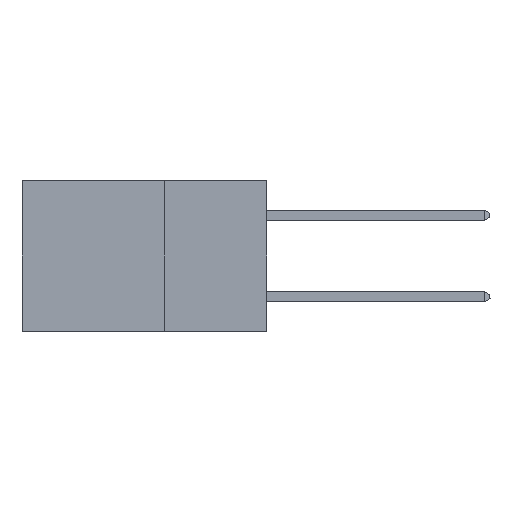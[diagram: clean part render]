
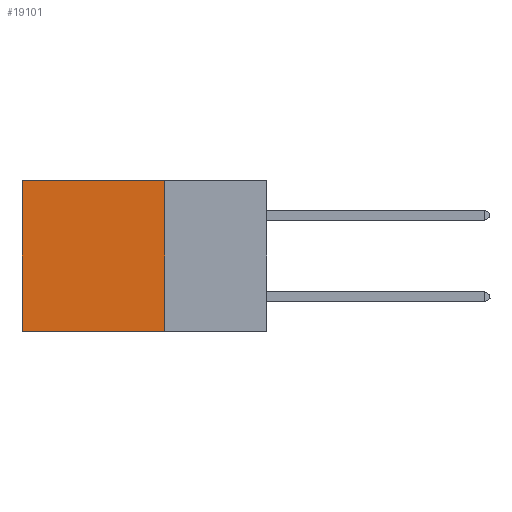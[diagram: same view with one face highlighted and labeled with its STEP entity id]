
A CAD part, left-side view. The second image highlights one B-rep face of the part: STEP entity #19101.
In plain terms, the highlighted planar face has unit normal (-1, 0, 0).
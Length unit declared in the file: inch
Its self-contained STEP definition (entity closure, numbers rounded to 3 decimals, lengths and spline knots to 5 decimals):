
#28 = DIRECTION ( 'NONE',  ( 0., 1., 0. ) ) ;
#558 = ORIENTED_EDGE ( 'NONE', *, *, #1156, .T. ) ;
#1156 = EDGE_CURVE ( 'NONE', #19799, #18990, #14665, .T. ) ;
#2888 = CARTESIAN_POINT ( 'NONE',  ( 0.2875, 0.25, 0. ) ) ;
#3376 = DIRECTION ( 'NONE',  ( 0., 1., 0. ) ) ;
#3559 = CARTESIAN_POINT ( 'NONE',  ( 0.2875, 0.25, 0. ) ) ;
#3904 = VECTOR ( 'NONE', #14393, 39.37008 ) ;
#3976 = VECTOR ( 'NONE', #3376, 39.37008 ) ;
#7139 = ORIENTED_EDGE ( 'NONE', *, *, #22710, .T. ) ;
#7356 = CARTESIAN_POINT ( 'NONE',  ( 0.2875, 0.6, -0.37 ) ) ;
#7572 = AXIS2_PLACEMENT_3D ( 'NONE', #2888, #20897, #8962 ) ;
#8962 = DIRECTION ( 'NONE',  ( 0., 0., -1. ) ) ;
#10166 = EDGE_LOOP ( 'NONE', ( #7139, #22189, #18478, #558 ) ) ;
#11651 = DIRECTION ( 'NONE',  ( 0., 0., -1. ) ) ;
#12366 = CARTESIAN_POINT ( 'NONE',  ( 0.2875, 0.6, 0. ) ) ;
#14393 = DIRECTION ( 'NONE',  ( 0., 0., -1. ) ) ;
#14583 = LINE ( 'NONE', #21524, #19847 ) ;
#14604 = CARTESIAN_POINT ( 'NONE',  ( 0.2875, 0.6, 0. ) ) ;
#14665 = LINE ( 'NONE', #3559, #3976 ) ;
#14935 = PLANE ( 'NONE',  #7572 ) ;
#15094 = VERTEX_POINT ( 'NONE', #7356 ) ;
#16338 = FACE_OUTER_BOUND ( 'NONE', #10166, .T. ) ;
#16827 = VERTEX_POINT ( 'NONE', #25255 ) ;
#16915 = LINE ( 'NONE', #24041, #20905 ) ;
#18478 = ORIENTED_EDGE ( 'NONE', *, *, #23119, .F. ) ;
#18990 = VERTEX_POINT ( 'NONE', #14604 ) ;
#19101 = ADVANCED_FACE ( 'NONE', ( #16338 ), #14935, .F. ) ;
#19531 = EDGE_CURVE ( 'NONE', #16827, #15094, #16915, .T. ) ;
#19799 = VERTEX_POINT ( 'NONE', #24608 ) ;
#19847 = VECTOR ( 'NONE', #11651, 39.37008 ) ;
#19869 = LINE ( 'NONE', #12366, #3904 ) ;
#20897 = DIRECTION ( 'NONE',  ( 1., 0., 0. ) ) ;
#20905 = VECTOR ( 'NONE', #28, 39.37008 ) ;
#21524 = CARTESIAN_POINT ( 'NONE',  ( 0.2875, 0.25, 0. ) ) ;
#22189 = ORIENTED_EDGE ( 'NONE', *, *, #19531, .F. ) ;
#22710 = EDGE_CURVE ( 'NONE', #18990, #15094, #19869, .T. ) ;
#23119 = EDGE_CURVE ( 'NONE', #19799, #16827, #14583, .T. ) ;
#24041 = CARTESIAN_POINT ( 'NONE',  ( 0.2875, 0.25, -0.37 ) ) ;
#24608 = CARTESIAN_POINT ( 'NONE',  ( 0.2875, 0.25, 0. ) ) ;
#25255 = CARTESIAN_POINT ( 'NONE',  ( 0.2875, 0.25, -0.37 ) ) ;
